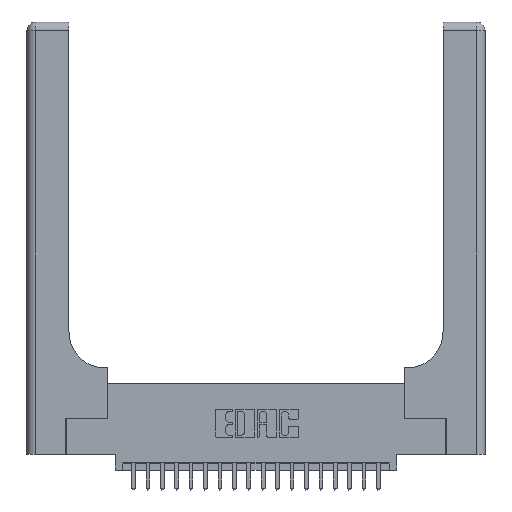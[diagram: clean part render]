
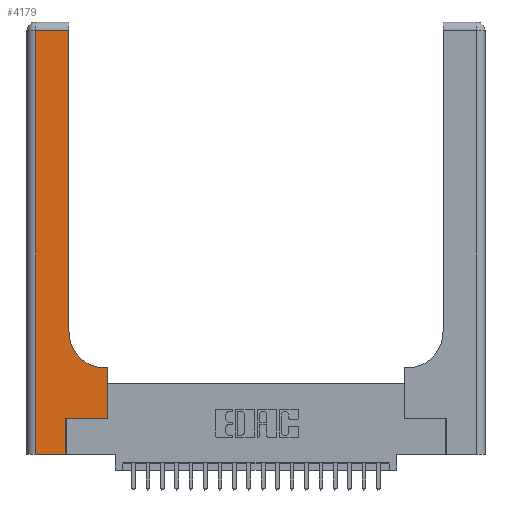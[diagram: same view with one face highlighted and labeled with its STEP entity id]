
A CAD part, top view. The second image highlights one B-rep face of the part: STEP entity #4179.
In plain terms, the highlighted planar face has unit normal (0, 0, 1).
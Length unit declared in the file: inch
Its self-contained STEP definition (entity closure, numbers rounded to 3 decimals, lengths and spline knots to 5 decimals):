
#465 = VECTOR ( 'NONE', #12322, 39.37008 ) ;
#510 = VERTEX_POINT ( 'NONE', #21178 ) ;
#684 = CARTESIAN_POINT ( 'NONE',  ( 0.269, 0.25, 0.37 ) ) ;
#701 = CARTESIAN_POINT ( 'NONE',  ( 0.06, 3., 0.37 ) ) ;
#737 = ORIENTED_EDGE ( 'NONE', *, *, #12523, .T. ) ;
#1192 = DIRECTION ( 'NONE',  ( 0., 1., 0. ) ) ;
#1306 = VERTEX_POINT ( 'NONE', #684 ) ;
#2129 = LINE ( 'NONE', #15152, #19688 ) ;
#2243 = EDGE_CURVE ( 'NONE', #17386, #14778, #9796, .T. ) ;
#2825 = VECTOR ( 'NONE', #3523, 39.37008 ) ;
#2862 = EDGE_CURVE ( 'NONE', #510, #11399, #2129, .T. ) ;
#3025 = CARTESIAN_POINT ( 'NONE',  ( 0.2915, 3., 0.37 ) ) ;
#3141 = DIRECTION ( 'NONE',  ( 1., 0., 0. ) ) ;
#3148 = FACE_OUTER_BOUND ( 'NONE', #11404, .T. ) ;
#3348 = CARTESIAN_POINT ( 'NONE',  ( 0.5415, 0.6, 0.37 ) ) ;
#3470 = EDGE_CURVE ( 'NONE', #16883, #17386, #18828, .T. ) ;
#3523 = DIRECTION ( 'NONE',  ( 0., 1., 0. ) ) ;
#3599 = LINE ( 'NONE', #4794, #7997 ) ;
#4179 = ADVANCED_FACE ( 'NONE', ( #3148 ), #6927, .F. ) ;
#4421 = CARTESIAN_POINT ( 'NONE',  ( 0.06, 0., 0.37 ) ) ;
#4653 = VECTOR ( 'NONE', #10196, 39.37008 ) ;
#4794 = CARTESIAN_POINT ( 'NONE',  ( 0., 0., 0.37 ) ) ;
#5421 = AXIS2_PLACEMENT_3D ( 'NONE', #10944, #14058, #17938 ) ;
#5812 = CARTESIAN_POINT ( 'NONE',  ( 0.2915, 0.85, 0.37 ) ) ;
#5933 = CARTESIAN_POINT ( 'NONE',  ( 0.06, 2.94, 0.37 ) ) ;
#5974 = LINE ( 'NONE', #701, #6521 ) ;
#6466 = VECTOR ( 'NONE', #1192, 39.37008 ) ;
#6521 = VECTOR ( 'NONE', #14690, 39.37008 ) ;
#6725 = CARTESIAN_POINT ( 'NONE',  ( 0.5585, 0.25, 0.37 ) ) ;
#6927 = PLANE ( 'NONE',  #19091 ) ;
#6987 = EDGE_CURVE ( 'NONE', #7996, #1306, #15875, .T. ) ;
#7570 = ORIENTED_EDGE ( 'NONE', *, *, #6987, .T. ) ;
#7843 = ORIENTED_EDGE ( 'NONE', *, *, #15385, .T. ) ;
#7889 = CARTESIAN_POINT ( 'NONE',  ( 0.269, 0., 0.37 ) ) ;
#7996 = VERTEX_POINT ( 'NONE', #17100 ) ;
#7997 = VECTOR ( 'NONE', #16982, 39.37008 ) ;
#9796 = CIRCLE ( 'NONE', #5421, 0.25 ) ;
#9845 = VERTEX_POINT ( 'NONE', #4421 ) ;
#10196 = DIRECTION ( 'NONE',  ( 0., 1., 0. ) ) ;
#10210 = CARTESIAN_POINT ( 'NONE',  ( 0.2915, 0.6, 0.37 ) ) ;
#10944 = CARTESIAN_POINT ( 'NONE',  ( 0.5415, 0.85, 0.37 ) ) ;
#11399 = VERTEX_POINT ( 'NONE', #5933 ) ;
#11404 = EDGE_LOOP ( 'NONE', ( #12881, #11792, #21986, #7843, #7570, #737, #12204, #18448, #12549 ) ) ;
#11572 = CARTESIAN_POINT ( 'NONE',  ( 0.269, 0.25, 0.37 ) ) ;
#11668 = LINE ( 'NONE', #3025, #6466 ) ;
#11792 = ORIENTED_EDGE ( 'NONE', *, *, #2862, .T. ) ;
#12204 = ORIENTED_EDGE ( 'NONE', *, *, #19927, .T. ) ;
#12276 = DIRECTION ( 'NONE',  ( -1., 0., 0. ) ) ;
#12322 = DIRECTION ( 'NONE',  ( -1., 0., 0. ) ) ;
#12523 = EDGE_CURVE ( 'NONE', #1306, #14094, #21539, .T. ) ;
#12549 = ORIENTED_EDGE ( 'NONE', *, *, #2243, .T. ) ;
#12881 = ORIENTED_EDGE ( 'NONE', *, *, #18538, .T. ) ;
#14058 = DIRECTION ( 'NONE',  ( 0., 0., -1. ) ) ;
#14094 = VERTEX_POINT ( 'NONE', #6725 ) ;
#14690 = DIRECTION ( 'NONE',  ( 0., -1., 0. ) ) ;
#14778 = VERTEX_POINT ( 'NONE', #5812 ) ;
#15152 = CARTESIAN_POINT ( 'NONE',  ( 0., 2.94, 0.37 ) ) ;
#15385 = EDGE_CURVE ( 'NONE', #9845, #7996, #3599, .T. ) ;
#15442 = CARTESIAN_POINT ( 'NONE',  ( 0.5585, 0.6, 0.37 ) ) ;
#15645 = CARTESIAN_POINT ( 'NONE',  ( 0., 3., 0.37 ) ) ;
#15875 = LINE ( 'NONE', #7889, #4653 ) ;
#16804 = LINE ( 'NONE', #17491, #2825 ) ;
#16883 = VERTEX_POINT ( 'NONE', #15442 ) ;
#16982 = DIRECTION ( 'NONE',  ( 1., 0., 0. ) ) ;
#17100 = CARTESIAN_POINT ( 'NONE',  ( 0.269, 0., 0.37 ) ) ;
#17386 = VERTEX_POINT ( 'NONE', #3348 ) ;
#17491 = CARTESIAN_POINT ( 'NONE',  ( 0.5585, 0.25, 0.37 ) ) ;
#17600 = DIRECTION ( 'NONE',  ( 0., 0., -1. ) ) ;
#17733 = VECTOR ( 'NONE', #3141, 39.37008 ) ;
#17826 = EDGE_CURVE ( 'NONE', #11399, #9845, #5974, .T. ) ;
#17938 = DIRECTION ( 'NONE',  ( 1., 0., 0. ) ) ;
#18448 = ORIENTED_EDGE ( 'NONE', *, *, #3470, .T. ) ;
#18538 = EDGE_CURVE ( 'NONE', #14778, #510, #11668, .T. ) ;
#18828 = LINE ( 'NONE', #10210, #465 ) ;
#19091 = AXIS2_PLACEMENT_3D ( 'NONE', #15645, #17600, #12276 ) ;
#19688 = VECTOR ( 'NONE', #22128, 39.37008 ) ;
#19927 = EDGE_CURVE ( 'NONE', #14094, #16883, #16804, .T. ) ;
#21178 = CARTESIAN_POINT ( 'NONE',  ( 0.2915, 2.94, 0.37 ) ) ;
#21539 = LINE ( 'NONE', #11572, #17733 ) ;
#21986 = ORIENTED_EDGE ( 'NONE', *, *, #17826, .T. ) ;
#22128 = DIRECTION ( 'NONE',  ( -1., 0., 0. ) ) ;
